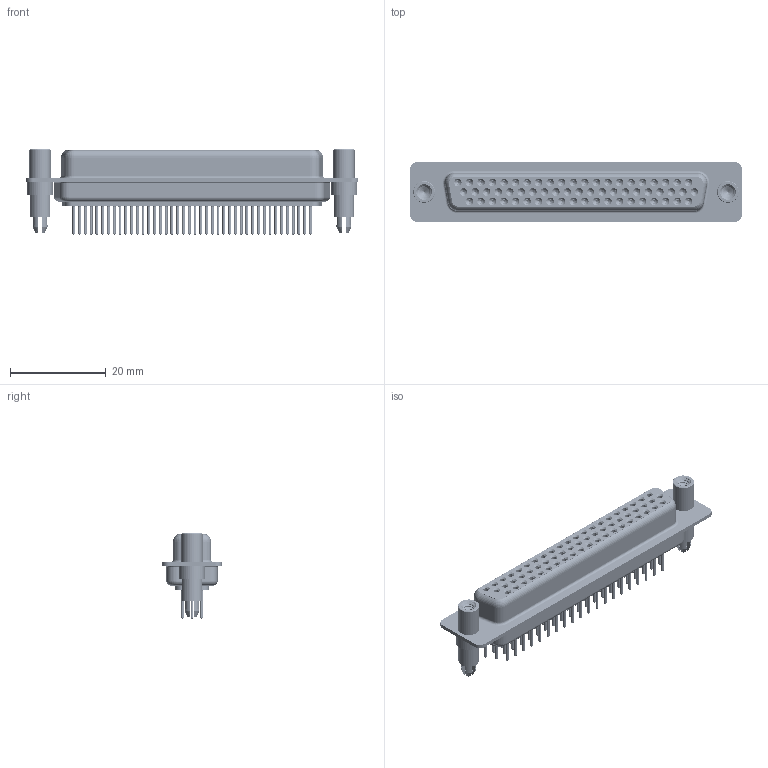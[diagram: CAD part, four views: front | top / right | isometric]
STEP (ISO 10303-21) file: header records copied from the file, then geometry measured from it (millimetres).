
FILE_DESCRIPTION (( 'STEP AP203' ), '1' );
FILE_NAME ('638-M62-330-BT6.STEP', '2022-07-05T21:34:48', ( '' ), ( '' ), 'SwSTEP 2.0', 'SolidWorks 2020', '' );
FILE_SCHEMA (( 'CONFIG_CONTROL_DESIGN' ));
Length unit declared in the file: millimetre
Products named in the file (8): 638M Housing_62 Contacts; 638M Contact Row 1_30; 638-M62-330-BT6; 638M Shell Front_62 Contacts; 638M Contact Row 2_30; 638M Shell Rear_62 Contacts; 638M 4-40 Threaded Standoff and Boardlock; 638M Contact Row 3_30
Assembly tree (67 placements, depth 2):
  638-M62-330-BT6
    638M Housing_62 Contacts
    638M Shell Front_62 Contacts
    638M Shell Rear_62 Contacts
    638M Contact Row 1_30  x21
    638M Contact Row 2_30  x21
    638M Contact Row 3_30  x20
    638M 4-40 Threaded Standoff and Boardlock  x2
Bounding box: 69.4 x 12.5 x 17.8 mm (x, y, z)
Volume: 5318.7 mm3; surface area: 16924.4 mm2
Topology: 67 solids, 67 shells, 3773 faces, 8709 edges, 5339 vertices
Faces by surface type: cylinder 1351, plane 1035, torus 925, cone 456, bspline 6
Entity records: 38577 total; most frequent: CARTESIAN_POINT 7173, DIRECTION 6785, ORIENTED_EDGE 5464, AXIS2_PLACEMENT_3D 2888, EDGE_CURVE 2732, VERTEX_POINT 1737, CIRCLE 1601, EDGE_LOOP 1567
